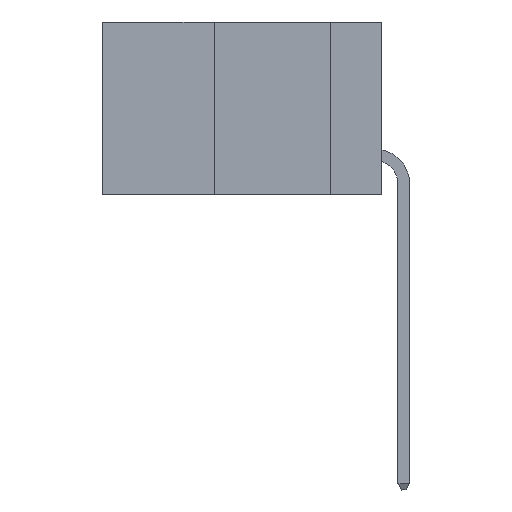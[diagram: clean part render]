
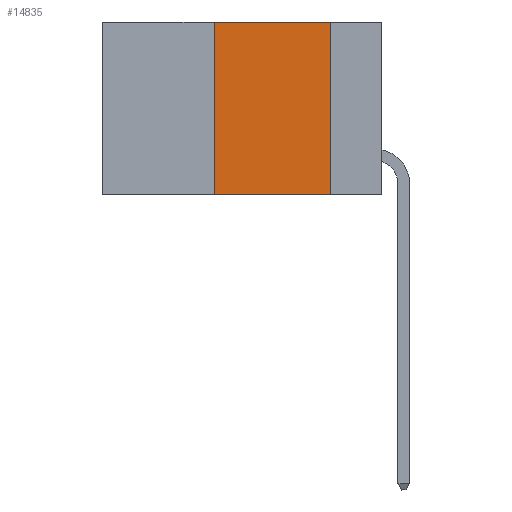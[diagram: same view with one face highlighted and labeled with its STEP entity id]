
A CAD part, left-side view. The second image highlights one B-rep face of the part: STEP entity #14835.
In plain terms, the highlighted planar face has unit normal (-1, 0, 0).
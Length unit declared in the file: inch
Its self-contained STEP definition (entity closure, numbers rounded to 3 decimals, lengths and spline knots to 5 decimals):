
#217 = CARTESIAN_POINT ( 'NONE',  ( 0., 0.11, -0.37 ) ) ;
#623 = EDGE_CURVE ( 'NONE', #2842, #22692, #2882, .T. ) ;
#677 = EDGE_CURVE ( 'NONE', #21855, #1551, #20771, .T. ) ;
#1016 = EDGE_CURVE ( 'NONE', #1551, #22692, #10708, .T. ) ;
#1041 = AXIS2_PLACEMENT_3D ( 'NONE', #9267, #18631, #16606 ) ;
#1551 = VERTEX_POINT ( 'NONE', #5716 ) ;
#2842 = VERTEX_POINT ( 'NONE', #5450 ) ;
#2882 = LINE ( 'NONE', #21633, #19948 ) ;
#3182 = LINE ( 'NONE', #17806, #6808 ) ;
#5450 = CARTESIAN_POINT ( 'NONE',  ( 0., 0.36, -0.37 ) ) ;
#5716 = CARTESIAN_POINT ( 'NONE',  ( 0., 0.11, 0. ) ) ;
#5921 = VECTOR ( 'NONE', #13663, 39.37008 ) ;
#6808 = VECTOR ( 'NONE', #21180, 39.37008 ) ;
#9035 = PLANE ( 'NONE',  #1041 ) ;
#9267 = CARTESIAN_POINT ( 'NONE',  ( 0., 0.6, 0. ) ) ;
#9696 = FACE_OUTER_BOUND ( 'NONE', #12140, .T. ) ;
#10063 = CARTESIAN_POINT ( 'NONE',  ( 0., 0.11, 0. ) ) ;
#10708 = LINE ( 'NONE', #10063, #5921 ) ;
#10986 = DIRECTION ( 'NONE',  ( 0., -1., 0. ) ) ;
#12140 = EDGE_LOOP ( 'NONE', ( #21152, #16724, #17215, #17124 ) ) ;
#13663 = DIRECTION ( 'NONE',  ( 0., 0., -1. ) ) ;
#14835 = ADVANCED_FACE ( 'NONE', ( #9696 ), #9035, .F. ) ;
#16167 = DIRECTION ( 'NONE',  ( 0., -1., 0. ) ) ;
#16606 = DIRECTION ( 'NONE',  ( 0., 0., -1. ) ) ;
#16724 = ORIENTED_EDGE ( 'NONE', *, *, #677, .F. ) ;
#17124 = ORIENTED_EDGE ( 'NONE', *, *, #623, .T. ) ;
#17215 = ORIENTED_EDGE ( 'NONE', *, *, #17341, .F. ) ;
#17341 = EDGE_CURVE ( 'NONE', #2842, #21855, #3182, .T. ) ;
#17806 = CARTESIAN_POINT ( 'NONE',  ( 0., 0.36, 0. ) ) ;
#17950 = CARTESIAN_POINT ( 'NONE',  ( 0., 0.6, 0. ) ) ;
#18631 = DIRECTION ( 'NONE',  ( 1., 0., 0. ) ) ;
#18803 = CARTESIAN_POINT ( 'NONE',  ( 0., 0.36, 0. ) ) ;
#19948 = VECTOR ( 'NONE', #16167, 39.37008 ) ;
#20771 = LINE ( 'NONE', #17950, #22746 ) ;
#21152 = ORIENTED_EDGE ( 'NONE', *, *, #1016, .F. ) ;
#21180 = DIRECTION ( 'NONE',  ( 0., 0., 1. ) ) ;
#21633 = CARTESIAN_POINT ( 'NONE',  ( 0., 0.6, -0.37 ) ) ;
#21855 = VERTEX_POINT ( 'NONE', #18803 ) ;
#22692 = VERTEX_POINT ( 'NONE', #217 ) ;
#22746 = VECTOR ( 'NONE', #10986, 39.37008 ) ;
